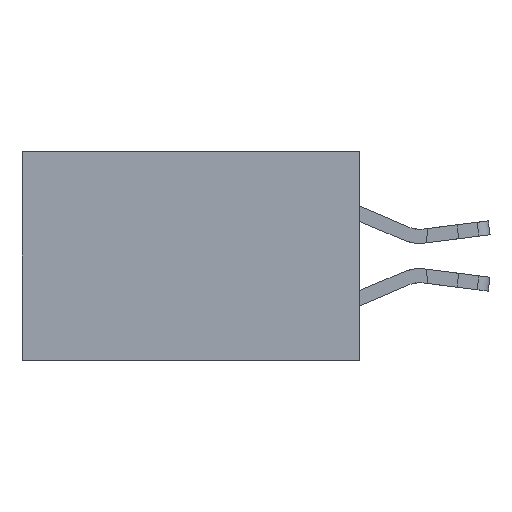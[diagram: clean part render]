
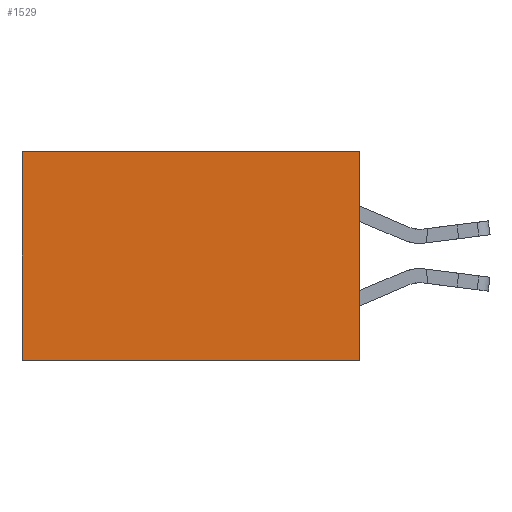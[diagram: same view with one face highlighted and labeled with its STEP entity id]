
A CAD part, left-side view. The second image highlights one B-rep face of the part: STEP entity #1529.
In plain terms, the highlighted planar face has unit normal (-1, 0, 0).
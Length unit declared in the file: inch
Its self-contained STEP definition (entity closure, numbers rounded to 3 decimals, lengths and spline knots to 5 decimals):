
#702 = ORIENTED_EDGE ( 'NONE', *, *, #14323, .T. ) ;
#763 = VERTEX_POINT ( 'NONE', #4176 ) ;
#810 = DIRECTION ( 'NONE',  ( 0., 0., -1. ) ) ;
#1529 = ADVANCED_FACE ( 'NONE', ( #17956 ), #2368, .F. ) ;
#2266 = VERTEX_POINT ( 'NONE', #20250 ) ;
#2368 = PLANE ( 'NONE',  #21169 ) ;
#3185 = CARTESIAN_POINT ( 'NONE',  ( 0.2875, 0., 0. ) ) ;
#3829 = EDGE_CURVE ( 'NONE', #7926, #11844, #9880, .T. ) ;
#4176 = CARTESIAN_POINT ( 'NONE',  ( 0.2875, 0.6, -0.37 ) ) ;
#4692 = ORIENTED_EDGE ( 'NONE', *, *, #3829, .F. ) ;
#5460 = CARTESIAN_POINT ( 'NONE',  ( 0.2875, 0., 0. ) ) ;
#5920 = VECTOR ( 'NONE', #18548, 39.37008 ) ;
#6638 = CARTESIAN_POINT ( 'NONE',  ( 0.2875, 0., 0. ) ) ;
#7256 = CARTESIAN_POINT ( 'NONE',  ( 0.2875, 0., -0.37 ) ) ;
#7926 = VERTEX_POINT ( 'NONE', #6638 ) ;
#8902 = EDGE_LOOP ( 'NONE', ( #17028, #12277, #4692, #702 ) ) ;
#9178 = DIRECTION ( 'NONE',  ( 0., 0., -1. ) ) ;
#9620 = LINE ( 'NONE', #14455, #12712 ) ;
#9880 = LINE ( 'NONE', #3185, #15548 ) ;
#10642 = DIRECTION ( 'NONE',  ( 1., 0., 0. ) ) ;
#10886 = CARTESIAN_POINT ( 'NONE',  ( 0.2875, 0.6, 0. ) ) ;
#11077 = EDGE_CURVE ( 'NONE', #2266, #763, #17214, .T. ) ;
#11844 = VERTEX_POINT ( 'NONE', #7256 ) ;
#12277 = ORIENTED_EDGE ( 'NONE', *, *, #16803, .F. ) ;
#12712 = VECTOR ( 'NONE', #21070, 39.37008 ) ;
#14323 = EDGE_CURVE ( 'NONE', #7926, #2266, #18739, .T. ) ;
#14455 = CARTESIAN_POINT ( 'NONE',  ( 0.2875, 0., -0.37 ) ) ;
#15548 = VECTOR ( 'NONE', #20935, 39.37008 ) ;
#16803 = EDGE_CURVE ( 'NONE', #11844, #763, #9620, .T. ) ;
#17028 = ORIENTED_EDGE ( 'NONE', *, *, #11077, .T. ) ;
#17214 = LINE ( 'NONE', #10886, #19744 ) ;
#17956 = FACE_OUTER_BOUND ( 'NONE', #8902, .T. ) ;
#18548 = DIRECTION ( 'NONE',  ( 0., 1., 0. ) ) ;
#18739 = LINE ( 'NONE', #5460, #5920 ) ;
#18832 = CARTESIAN_POINT ( 'NONE',  ( 0.2875, 0., 0. ) ) ;
#19744 = VECTOR ( 'NONE', #9178, 39.37008 ) ;
#20250 = CARTESIAN_POINT ( 'NONE',  ( 0.2875, 0.6, 0. ) ) ;
#20935 = DIRECTION ( 'NONE',  ( 0., 0., -1. ) ) ;
#21070 = DIRECTION ( 'NONE',  ( 0., 1., 0. ) ) ;
#21169 = AXIS2_PLACEMENT_3D ( 'NONE', #18832, #10642, #810 ) ;
